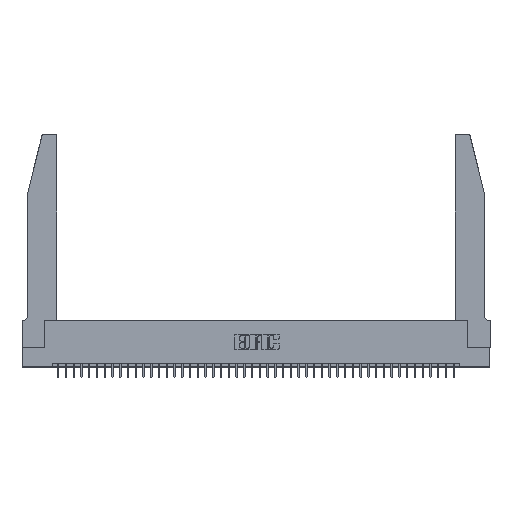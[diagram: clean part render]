
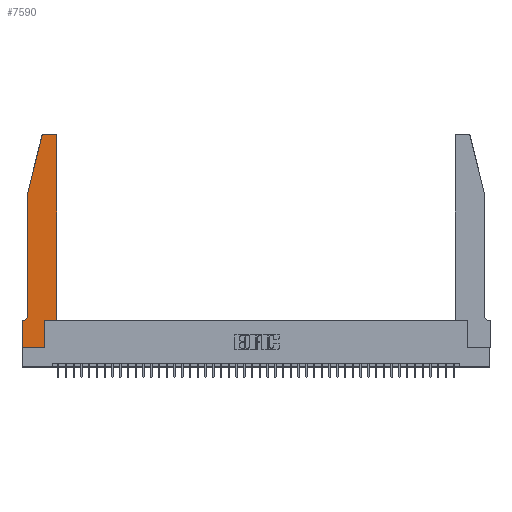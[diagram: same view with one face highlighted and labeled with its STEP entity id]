
A CAD part, top view. The second image highlights one B-rep face of the part: STEP entity #7590.
In plain terms, the highlighted planar face has unit normal (0, 0, 1).
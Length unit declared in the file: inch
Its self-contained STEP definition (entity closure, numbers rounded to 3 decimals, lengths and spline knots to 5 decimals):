
#1295 = ORIENTED_EDGE ( 'NONE', *, *, #43027, .T. ) ;
#1639 = DIRECTION ( 'NONE',  ( -1., 0., 0. ) ) ;
#1653 = VERTEX_POINT ( 'NONE', #3784 ) ;
#1758 = VECTOR ( 'NONE', #9984, 39.37008 ) ;
#2184 = CARTESIAN_POINT ( 'NONE',  ( 0.4505, 0.35, 0.37 ) ) ;
#3032 = LINE ( 'NONE', #40278, #37516 ) ;
#3751 = CARTESIAN_POINT ( 'NONE',  ( 0.4505, 2.72, 0.37 ) ) ;
#3784 = CARTESIAN_POINT ( 'NONE',  ( 0.25487, 2.72718, 0.37 ) ) ;
#4197 = AXIS2_PLACEMENT_3D ( 'NONE', #4294, #31910, #7916 ) ;
#4294 = CARTESIAN_POINT ( 'NONE',  ( 0.4205, 2.72, 0.37 ) ) ;
#4544 = AXIS2_PLACEMENT_3D ( 'NONE', #33521, #16002, #23655 ) ;
#5202 = EDGE_CURVE ( 'NONE', #36734, #25473, #3032, .T. ) ;
#6078 = AXIS2_PLACEMENT_3D ( 'NONE', #28126, #24761, #38409 ) ;
#7356 = VERTEX_POINT ( 'NONE', #23004 ) ;
#7590 = ADVANCED_FACE ( 'NONE', ( #10409 ), #18235, .T. ) ;
#7667 = VERTEX_POINT ( 'NONE', #32615 ) ;
#7916 = DIRECTION ( 'NONE',  ( 1., 0., 0. ) ) ;
#8246 = EDGE_CURVE ( 'NONE', #19376, #35213, #43501, .T. ) ;
#8973 = CARTESIAN_POINT ( 'NONE',  ( 0., 0., 0.37 ) ) ;
#9572 = DIRECTION ( 'NONE',  ( -1., 0., 0. ) ) ;
#9647 = EDGE_CURVE ( 'NONE', #7667, #7356, #24449, .T. ) ;
#9984 = DIRECTION ( 'NONE',  ( 0., 1., 0. ) ) ;
#10204 = CARTESIAN_POINT ( 'NONE',  ( 0.2865, 0.35, 0.37 ) ) ;
#10323 = DIRECTION ( 'NONE',  ( -0.239, -0.971, 0. ) ) ;
#10409 = FACE_OUTER_BOUND ( 'NONE', #34188, .T. ) ;
#11786 = CARTESIAN_POINT ( 'NONE',  ( 0.0055, 0.42, 0.37 ) ) ;
#11878 = VECTOR ( 'NONE', #30306, 39.37008 ) ;
#13229 = ORIENTED_EDGE ( 'NONE', *, *, #14325, .T. ) ;
#13485 = CARTESIAN_POINT ( 'NONE',  ( 0.0755, 2., 0.37 ) ) ;
#13512 = CARTESIAN_POINT ( 'NONE',  ( 0.284, 2.75, 0.37 ) ) ;
#13923 = EDGE_CURVE ( 'NONE', #7356, #37487, #34813, .T. ) ;
#14325 = EDGE_CURVE ( 'NONE', #24231, #40101, #38552, .T. ) ;
#14365 = ORIENTED_EDGE ( 'NONE', *, *, #38200, .T. ) ;
#15382 = LINE ( 'NONE', #29542, #38684 ) ;
#16002 = DIRECTION ( 'NONE',  ( 0., 0., 1. ) ) ;
#16911 = LINE ( 'NONE', #10204, #1758 ) ;
#17291 = ORIENTED_EDGE ( 'NONE', *, *, #30557, .T. ) ;
#18235 = PLANE ( 'NONE',  #6078 ) ;
#19372 = ORIENTED_EDGE ( 'NONE', *, *, #9647, .T. ) ;
#19376 = VERTEX_POINT ( 'NONE', #34833 ) ;
#20495 = VECTOR ( 'NONE', #31404, 39.37008 ) ;
#21023 = CARTESIAN_POINT ( 'NONE',  ( 0.2865, 0.35, 0.37 ) ) ;
#21071 = CARTESIAN_POINT ( 'NONE',  ( 0.4505, 0.35, 0.37 ) ) ;
#21362 = EDGE_CURVE ( 'NONE', #1653, #7667, #37878, .T. ) ;
#22938 = ORIENTED_EDGE ( 'NONE', *, *, #42454, .T. ) ;
#23004 = CARTESIAN_POINT ( 'NONE',  ( 0.0755, 0.42, 0.37 ) ) ;
#23609 = CIRCLE ( 'NONE', #4197, 0.03 ) ;
#23655 = DIRECTION ( 'NONE',  ( 1., 0., 0. ) ) ;
#24213 = CARTESIAN_POINT ( 'NONE',  ( 0.0055, 0.35, 0.37 ) ) ;
#24231 = VERTEX_POINT ( 'NONE', #21023 ) ;
#24449 = LINE ( 'NONE', #28241, #26996 ) ;
#24761 = DIRECTION ( 'NONE',  ( 0., 0., 1. ) ) ;
#25224 = CARTESIAN_POINT ( 'NONE',  ( 0.4205, 2.75, 0.37 ) ) ;
#25473 = VERTEX_POINT ( 'NONE', #13512 ) ;
#26218 = VECTOR ( 'NONE', #40916, 39.37008 ) ;
#26996 = VECTOR ( 'NONE', #30971, 39.37008 ) ;
#27731 = LINE ( 'NONE', #31300, #26218 ) ;
#28126 = CARTESIAN_POINT ( 'NONE',  ( 0., 0.35, 0.37 ) ) ;
#28241 = CARTESIAN_POINT ( 'NONE',  ( 0.0755, 2., 0.37 ) ) ;
#28249 = VECTOR ( 'NONE', #38105, 39.37008 ) ;
#28505 = ORIENTED_EDGE ( 'NONE', *, *, #8246, .T. ) ;
#28639 = DIRECTION ( 'NONE',  ( 0., 0., -1. ) ) ;
#28958 = CIRCLE ( 'NONE', #4544, 0.03 ) ;
#29394 = VECTOR ( 'NONE', #10323, 39.37008 ) ;
#29542 = CARTESIAN_POINT ( 'NONE',  ( 0.0755, 0.35, 0.37 ) ) ;
#30306 = DIRECTION ( 'NONE',  ( 1., 0., 0. ) ) ;
#30557 = EDGE_CURVE ( 'NONE', #41732, #19376, #27731, .T. ) ;
#30971 = DIRECTION ( 'NONE',  ( 0., -1., 0. ) ) ;
#31130 = CARTESIAN_POINT ( 'NONE',  ( 0., 0.35, 0.37 ) ) ;
#31300 = CARTESIAN_POINT ( 'NONE',  ( 0., 0., 0.37 ) ) ;
#31404 = DIRECTION ( 'NONE',  ( 1., 0., 0. ) ) ;
#31415 = CARTESIAN_POINT ( 'NONE',  ( 0.4505, 0.35, 0.37 ) ) ;
#31910 = DIRECTION ( 'NONE',  ( 0., 0., 1. ) ) ;
#32450 = DIRECTION ( 'NONE',  ( -1., 0., 0. ) ) ;
#32615 = CARTESIAN_POINT ( 'NONE',  ( 0.0755, 2., 0.37 ) ) ;
#32686 = ORIENTED_EDGE ( 'NONE', *, *, #5202, .T. ) ;
#33521 = CARTESIAN_POINT ( 'NONE',  ( 0.284, 2.72, 0.37 ) ) ;
#34161 = VERTEX_POINT ( 'NONE', #3751 ) ;
#34188 = EDGE_LOOP ( 'NONE', ( #32686, #22938, #37317, #19372, #40913, #14365, #17291, #28505, #43042, #13229, #1295, #37056 ) ) ;
#34813 = CIRCLE ( 'NONE', #44090, 0.07 ) ;
#34833 = CARTESIAN_POINT ( 'NONE',  ( 0., 0., 0.37 ) ) ;
#35213 = VERTEX_POINT ( 'NONE', #38191 ) ;
#35491 = EDGE_CURVE ( 'NONE', #34161, #36734, #23609, .T. ) ;
#36734 = VERTEX_POINT ( 'NONE', #25224 ) ;
#37056 = ORIENTED_EDGE ( 'NONE', *, *, #35491, .T. ) ;
#37317 = ORIENTED_EDGE ( 'NONE', *, *, #21362, .T. ) ;
#37449 = LINE ( 'NONE', #31415, #28249 ) ;
#37487 = VERTEX_POINT ( 'NONE', #24213 ) ;
#37516 = VECTOR ( 'NONE', #9572, 39.37008 ) ;
#37878 = LINE ( 'NONE', #13485, #29394 ) ;
#38105 = DIRECTION ( 'NONE',  ( 0., 1., 0. ) ) ;
#38191 = CARTESIAN_POINT ( 'NONE',  ( 0.2865, 0., 0.37 ) ) ;
#38200 = EDGE_CURVE ( 'NONE', #37487, #41732, #15382, .T. ) ;
#38409 = DIRECTION ( 'NONE',  ( 1., 0., 0. ) ) ;
#38552 = LINE ( 'NONE', #21071, #20495 ) ;
#38684 = VECTOR ( 'NONE', #32450, 39.37008 ) ;
#40101 = VERTEX_POINT ( 'NONE', #2184 ) ;
#40278 = CARTESIAN_POINT ( 'NONE',  ( 0.2605, 2.75, 0.37 ) ) ;
#40913 = ORIENTED_EDGE ( 'NONE', *, *, #13923, .T. ) ;
#40916 = DIRECTION ( 'NONE',  ( 0., -1., 0. ) ) ;
#41732 = VERTEX_POINT ( 'NONE', #31130 ) ;
#42454 = EDGE_CURVE ( 'NONE', #25473, #1653, #28958, .T. ) ;
#43027 = EDGE_CURVE ( 'NONE', #40101, #34161, #37449, .T. ) ;
#43042 = ORIENTED_EDGE ( 'NONE', *, *, #43993, .T. ) ;
#43501 = LINE ( 'NONE', #8973, #11878 ) ;
#43993 = EDGE_CURVE ( 'NONE', #35213, #24231, #16911, .T. ) ;
#44090 = AXIS2_PLACEMENT_3D ( 'NONE', #11786, #28639, #1639 ) ;
